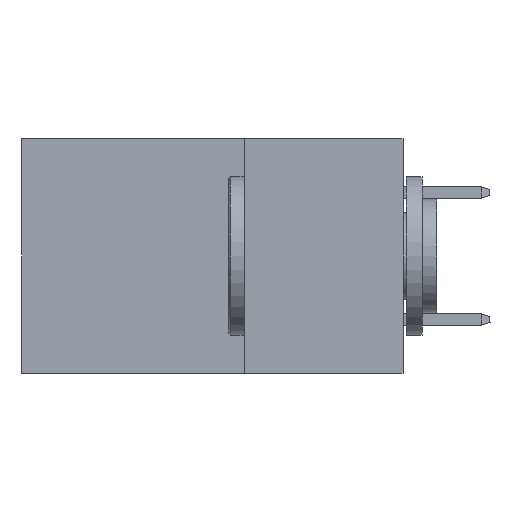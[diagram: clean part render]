
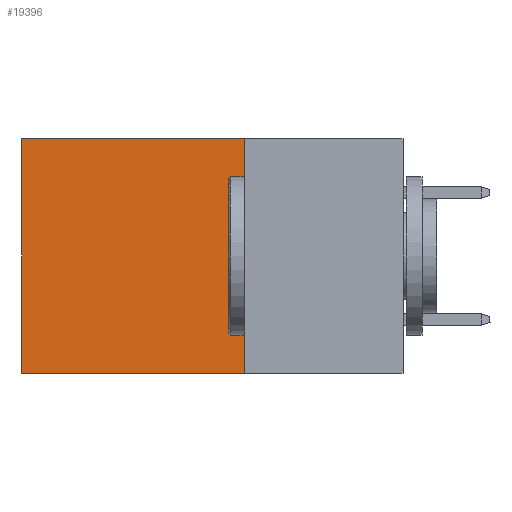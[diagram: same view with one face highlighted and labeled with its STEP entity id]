
A CAD part, left-side view. The second image highlights one B-rep face of the part: STEP entity #19396.
In plain terms, the highlighted planar face has unit normal (-1, 0, 0).
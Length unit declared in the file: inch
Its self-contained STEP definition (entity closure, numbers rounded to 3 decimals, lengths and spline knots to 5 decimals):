
#2197 = DIRECTION ( 'NONE',  ( 0., 0., -1. ) ) ;
#3391 = CARTESIAN_POINT ( 'NONE',  ( 0.2875, 0.6, -0.37 ) ) ;
#8242 = VECTOR ( 'NONE', #40398, 39.37008 ) ;
#8731 = CARTESIAN_POINT ( 'NONE',  ( 0.2875, 0.6, 0. ) ) ;
#8861 = ORIENTED_EDGE ( 'NONE', *, *, #34003, .T. ) ;
#9180 = VECTOR ( 'NONE', #30839, 39.37008 ) ;
#9997 = CARTESIAN_POINT ( 'NONE',  ( 0.2875, 0.25, 0. ) ) ;
#10393 = VERTEX_POINT ( 'NONE', #19394 ) ;
#12512 = LINE ( 'NONE', #8731, #23198 ) ;
#13809 = LINE ( 'NONE', #17587, #33465 ) ;
#14353 = VERTEX_POINT ( 'NONE', #42109 ) ;
#14422 = VERTEX_POINT ( 'NONE', #42343 ) ;
#17587 = CARTESIAN_POINT ( 'NONE',  ( 0.2875, 0.25, -0.37 ) ) ;
#18677 = EDGE_CURVE ( 'NONE', #10393, #14422, #21950, .T. ) ;
#19394 = CARTESIAN_POINT ( 'NONE',  ( 0.2875, 0.25, 0. ) ) ;
#19396 = ADVANCED_FACE ( 'NONE', ( #38168 ), #24660, .F. ) ;
#19739 = CARTESIAN_POINT ( 'NONE',  ( 0.2875, 0.25, 0. ) ) ;
#21950 = LINE ( 'NONE', #29498, #8242 ) ;
#23198 = VECTOR ( 'NONE', #42076, 39.37008 ) ;
#24087 = ORIENTED_EDGE ( 'NONE', *, *, #18677, .F. ) ;
#24660 = PLANE ( 'NONE',  #26423 ) ;
#25275 = EDGE_CURVE ( 'NONE', #14422, #31138, #13809, .T. ) ;
#26423 = AXIS2_PLACEMENT_3D ( 'NONE', #9997, #38396, #2197 ) ;
#28230 = DIRECTION ( 'NONE',  ( 0., 1., 0. ) ) ;
#29498 = CARTESIAN_POINT ( 'NONE',  ( 0.2875, 0.25, 0. ) ) ;
#30839 = DIRECTION ( 'NONE',  ( 0., 1., 0. ) ) ;
#31138 = VERTEX_POINT ( 'NONE', #3391 ) ;
#33465 = VECTOR ( 'NONE', #28230, 39.37008 ) ;
#34003 = EDGE_CURVE ( 'NONE', #10393, #14353, #38190, .T. ) ;
#37512 = ORIENTED_EDGE ( 'NONE', *, *, #25275, .F. ) ;
#37743 = ORIENTED_EDGE ( 'NONE', *, *, #41943, .T. ) ;
#38168 = FACE_OUTER_BOUND ( 'NONE', #43231, .T. ) ;
#38190 = LINE ( 'NONE', #19739, #9180 ) ;
#38396 = DIRECTION ( 'NONE',  ( 1., 0., 0. ) ) ;
#40398 = DIRECTION ( 'NONE',  ( 0., 0., -1. ) ) ;
#41943 = EDGE_CURVE ( 'NONE', #14353, #31138, #12512, .T. ) ;
#42076 = DIRECTION ( 'NONE',  ( 0., 0., -1. ) ) ;
#42109 = CARTESIAN_POINT ( 'NONE',  ( 0.2875, 0.6, 0. ) ) ;
#42343 = CARTESIAN_POINT ( 'NONE',  ( 0.2875, 0.25, -0.37 ) ) ;
#43231 = EDGE_LOOP ( 'NONE', ( #37743, #37512, #24087, #8861 ) ) ;
